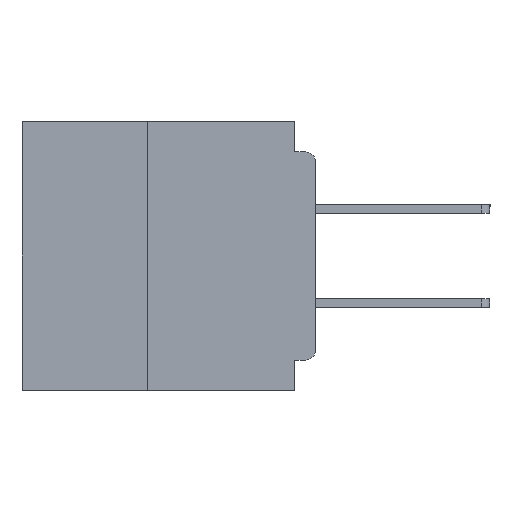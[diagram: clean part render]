
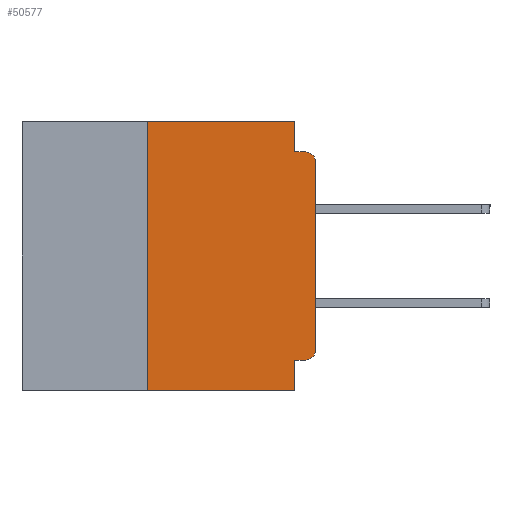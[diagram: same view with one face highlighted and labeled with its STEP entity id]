
A CAD part, left-side view. The second image highlights one B-rep face of the part: STEP entity #50577.
In plain terms, the highlighted planar face has unit normal (-1, 0, 0).
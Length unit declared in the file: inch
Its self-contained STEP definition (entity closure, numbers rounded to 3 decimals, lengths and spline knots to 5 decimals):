
#1675 = EDGE_CURVE ( 'NONE', #54785, #33096, #52505, .T. ) ;
#1870 = CARTESIAN_POINT ( 'NONE',  ( 0., 0.031, -0.4 ) ) ;
#2064 = DIRECTION ( 'NONE',  ( 0., 0., -1. ) ) ;
#2286 = ORIENTED_EDGE ( 'NONE', *, *, #1675, .F. ) ;
#5221 = ORIENTED_EDGE ( 'NONE', *, *, #14591, .F. ) ;
#5846 = LINE ( 'NONE', #49932, #29677 ) ;
#7661 = VERTEX_POINT ( 'NONE', #35658 ) ;
#8845 = LINE ( 'NONE', #11356, #57981 ) ;
#9888 = EDGE_CURVE ( 'NONE', #24182, #33096, #18568, .T. ) ;
#10118 = FACE_OUTER_BOUND ( 'NONE', #40526, .T. ) ;
#10251 = EDGE_CURVE ( 'NONE', #30088, #49175, #8845, .T. ) ;
#10501 = ORIENTED_EDGE ( 'NONE', *, *, #9888, .T. ) ;
#10526 = PLANE ( 'NONE',  #31581 ) ;
#10753 = CARTESIAN_POINT ( 'NONE',  ( 0., 0.437, 0. ) ) ;
#11107 = CARTESIAN_POINT ( 'NONE',  ( 0., 0., -0.34 ) ) ;
#11124 = ORIENTED_EDGE ( 'NONE', *, *, #10251, .F. ) ;
#11356 = CARTESIAN_POINT ( 'NONE',  ( 0., 0., -0.045 ) ) ;
#13305 = ORIENTED_EDGE ( 'NONE', *, *, #33613, .T. ) ;
#14003 = DIRECTION ( 'NONE',  ( -1., 0., 0. ) ) ;
#14221 = VECTOR ( 'NONE', #41030, 39.37008 ) ;
#14502 = VECTOR ( 'NONE', #2064, 39.37008 ) ;
#14591 = EDGE_CURVE ( 'NONE', #54733, #54785, #37366, .T. ) ;
#15084 = VECTOR ( 'NONE', #21056, 39.37008 ) ;
#15138 = CARTESIAN_POINT ( 'NONE',  ( 0., 0.031, 0. ) ) ;
#15518 = DIRECTION ( 'NONE',  ( 0., 0., -1. ) ) ;
#15703 = CARTESIAN_POINT ( 'NONE',  ( 0., 0.437, 0. ) ) ;
#16838 = DIRECTION ( 'NONE',  ( 0., 0., 1. ) ) ;
#17374 = CARTESIAN_POINT ( 'NONE',  ( 0., 0., 0. ) ) ;
#17389 = CARTESIAN_POINT ( 'NONE',  ( 0., 0.031, -0.355 ) ) ;
#18068 = VERTEX_POINT ( 'NONE', #36352 ) ;
#18568 = LINE ( 'NONE', #51557, #29740 ) ;
#19862 = CARTESIAN_POINT ( 'NONE',  ( 0., 0.015, -0.06 ) ) ;
#20889 = DIRECTION ( 'NONE',  ( 0., -1., 0. ) ) ;
#21056 = DIRECTION ( 'NONE',  ( 0., 1., 0. ) ) ;
#22065 = VECTOR ( 'NONE', #48988, 39.37008 ) ;
#22292 = ORIENTED_EDGE ( 'NONE', *, *, #22363, .F. ) ;
#22363 = EDGE_CURVE ( 'NONE', #46445, #18068, #23561, .T. ) ;
#23307 = CARTESIAN_POINT ( 'NONE',  ( 0., 0.25, -0.4 ) ) ;
#23561 = LINE ( 'NONE', #15703, #22065 ) ;
#24182 = VERTEX_POINT ( 'NONE', #23307 ) ;
#24646 = DIRECTION ( 'NONE',  ( 0., 0., -1. ) ) ;
#26806 = EDGE_CURVE ( 'NONE', #54733, #58555, #30505, .T. ) ;
#26834 = LINE ( 'NONE', #17374, #14221 ) ;
#29101 = EDGE_CURVE ( 'NONE', #18068, #30088, #52275, .T. ) ;
#29265 = CARTESIAN_POINT ( 'NONE',  ( 0., 0.031, -0.4 ) ) ;
#29483 = DIRECTION ( 'NONE',  ( 0., 0., -1. ) ) ;
#29677 = VECTOR ( 'NONE', #16838, 39.37008 ) ;
#29740 = VECTOR ( 'NONE', #46753, 39.37008 ) ;
#30088 = VERTEX_POINT ( 'NONE', #51902 ) ;
#30505 = CIRCLE ( 'NONE', #44042, 0.015 ) ;
#31313 = CARTESIAN_POINT ( 'NONE',  ( 0., 0.015, -0.355 ) ) ;
#31581 = AXIS2_PLACEMENT_3D ( 'NONE', #10753, #44000, #15518 ) ;
#33096 = VERTEX_POINT ( 'NONE', #29265 ) ;
#33613 = EDGE_CURVE ( 'NONE', #7661, #49175, #37464, .T. ) ;
#33960 = CARTESIAN_POINT ( 'NONE',  ( 0., 0.015, -0.045 ) ) ;
#34121 = ORIENTED_EDGE ( 'NONE', *, *, #58119, .T. ) ;
#35658 = CARTESIAN_POINT ( 'NONE',  ( 0., 0., -0.06 ) ) ;
#36352 = CARTESIAN_POINT ( 'NONE',  ( 0., 0.031, 0. ) ) ;
#37366 = LINE ( 'NONE', #49590, #15084 ) ;
#37464 = CIRCLE ( 'NONE', #60247, 0.015 ) ;
#39548 = VECTOR ( 'NONE', #29483, 39.37008 ) ;
#40526 = EDGE_LOOP ( 'NONE', ( #34121, #13305, #11124, #45360, #22292, #44698, #10501, #2286, #5221, #58834 ) ) ;
#41030 = DIRECTION ( 'NONE',  ( 0., 0., 1. ) ) ;
#42456 = CARTESIAN_POINT ( 'NONE',  ( 0., 0.015, -0.34 ) ) ;
#44000 = DIRECTION ( 'NONE',  ( 1., 0., 0. ) ) ;
#44042 = AXIS2_PLACEMENT_3D ( 'NONE', #42456, #14003, #47295 ) ;
#44698 = ORIENTED_EDGE ( 'NONE', *, *, #48807, .F. ) ;
#45360 = ORIENTED_EDGE ( 'NONE', *, *, #29101, .F. ) ;
#46445 = VERTEX_POINT ( 'NONE', #60949 ) ;
#46753 = DIRECTION ( 'NONE',  ( 0., -1., 0. ) ) ;
#47295 = DIRECTION ( 'NONE',  ( 0., 0., -1. ) ) ;
#48807 = EDGE_CURVE ( 'NONE', #24182, #46445, #5846, .T. ) ;
#48988 = DIRECTION ( 'NONE',  ( 0., -1., 0. ) ) ;
#49175 = VERTEX_POINT ( 'NONE', #33960 ) ;
#49590 = CARTESIAN_POINT ( 'NONE',  ( 0., 0., -0.355 ) ) ;
#49932 = CARTESIAN_POINT ( 'NONE',  ( 0., 0.25, -0.4 ) ) ;
#50577 = ADVANCED_FACE ( 'NONE', ( #10118 ), #10526, .F. ) ;
#51557 = CARTESIAN_POINT ( 'NONE',  ( 0., 0.437, -0.4 ) ) ;
#51902 = CARTESIAN_POINT ( 'NONE',  ( 0., 0.031, -0.045 ) ) ;
#52275 = LINE ( 'NONE', #15138, #39548 ) ;
#52505 = LINE ( 'NONE', #1870, #14502 ) ;
#53232 = DIRECTION ( 'NONE',  ( -1., 0., 0. ) ) ;
#54733 = VERTEX_POINT ( 'NONE', #31313 ) ;
#54785 = VERTEX_POINT ( 'NONE', #17389 ) ;
#57981 = VECTOR ( 'NONE', #20889, 39.37008 ) ;
#58119 = EDGE_CURVE ( 'NONE', #58555, #7661, #26834, .T. ) ;
#58555 = VERTEX_POINT ( 'NONE', #11107 ) ;
#58834 = ORIENTED_EDGE ( 'NONE', *, *, #26806, .T. ) ;
#60247 = AXIS2_PLACEMENT_3D ( 'NONE', #19862, #53232, #24646 ) ;
#60949 = CARTESIAN_POINT ( 'NONE',  ( 0., 0.25, 0. ) ) ;
